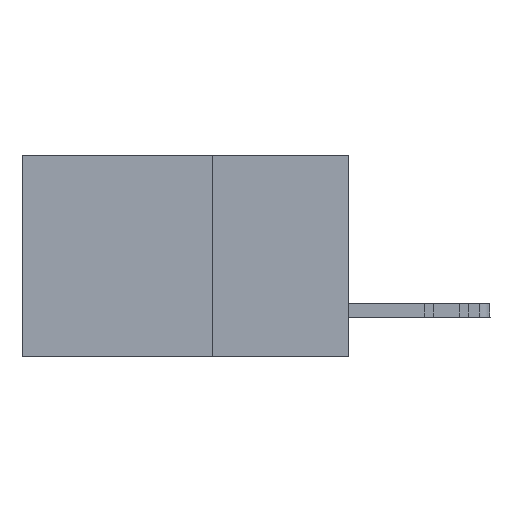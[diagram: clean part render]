
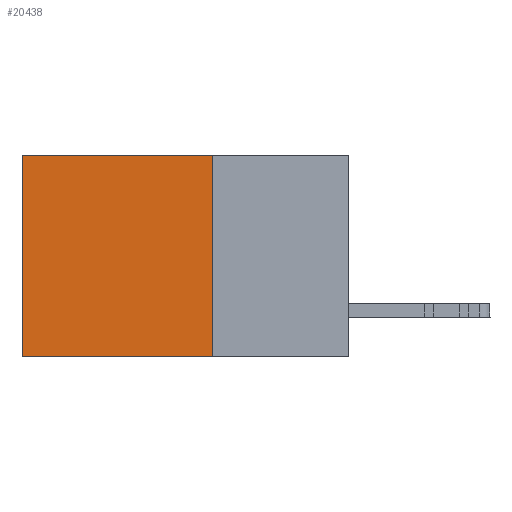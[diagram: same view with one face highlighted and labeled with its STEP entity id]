
A CAD part, left-side view. The second image highlights one B-rep face of the part: STEP entity #20438.
In plain terms, the highlighted planar face has unit normal (-1, 0, 0).
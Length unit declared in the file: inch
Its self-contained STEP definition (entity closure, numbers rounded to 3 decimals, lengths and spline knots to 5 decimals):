
#853 = ORIENTED_EDGE ( 'NONE', *, *, #7887, .F. ) ;
#2678 = VECTOR ( 'NONE', #27529, 39.37008 ) ;
#4890 = DIRECTION ( 'NONE',  ( 0., 0., -1. ) ) ;
#5564 = CARTESIAN_POINT ( 'NONE',  ( 0.298, 0.6, -0.37 ) ) ;
#6428 = VECTOR ( 'NONE', #21301, 39.37008 ) ;
#6734 = EDGE_CURVE ( 'NONE', #13923, #8608, #21188, .T. ) ;
#6937 = CARTESIAN_POINT ( 'NONE',  ( 0.298, 0.25, 0. ) ) ;
#7636 = VERTEX_POINT ( 'NONE', #16326 ) ;
#7887 = EDGE_CURVE ( 'NONE', #7636, #16645, #14452, .T. ) ;
#8142 = EDGE_CURVE ( 'NONE', #8608, #16645, #19667, .T. ) ;
#8325 = LINE ( 'NONE', #6937, #30068 ) ;
#8608 = VERTEX_POINT ( 'NONE', #23305 ) ;
#13923 = VERTEX_POINT ( 'NONE', #23910 ) ;
#14452 = LINE ( 'NONE', #25871, #25848 ) ;
#14478 = DIRECTION ( 'NONE',  ( 0., 1., 0. ) ) ;
#16326 = CARTESIAN_POINT ( 'NONE',  ( 0.298, 0.25, -0.37 ) ) ;
#16645 = VERTEX_POINT ( 'NONE', #5564 ) ;
#17936 = ORIENTED_EDGE ( 'NONE', *, *, #21636, .F. ) ;
#18665 = EDGE_LOOP ( 'NONE', ( #27851, #853, #17936, #24856 ) ) ;
#19285 = DIRECTION ( 'NONE',  ( 0., 0., -1. ) ) ;
#19667 = LINE ( 'NONE', #25021, #2678 ) ;
#20438 = ADVANCED_FACE ( 'NONE', ( #27948 ), #28565, .F. ) ;
#21188 = LINE ( 'NONE', #30538, #6428 ) ;
#21301 = DIRECTION ( 'NONE',  ( 0., 1., 0. ) ) ;
#21636 = EDGE_CURVE ( 'NONE', #13923, #7636, #8325, .T. ) ;
#23305 = CARTESIAN_POINT ( 'NONE',  ( 0.298, 0.6, 0. ) ) ;
#23864 = AXIS2_PLACEMENT_3D ( 'NONE', #28868, #26180, #19285 ) ;
#23910 = CARTESIAN_POINT ( 'NONE',  ( 0.298, 0.25, 0. ) ) ;
#24856 = ORIENTED_EDGE ( 'NONE', *, *, #6734, .T. ) ;
#25021 = CARTESIAN_POINT ( 'NONE',  ( 0.298, 0.6, 0. ) ) ;
#25848 = VECTOR ( 'NONE', #14478, 39.37008 ) ;
#25871 = CARTESIAN_POINT ( 'NONE',  ( 0.298, 0.25, -0.37 ) ) ;
#26180 = DIRECTION ( 'NONE',  ( 1., 0., 0. ) ) ;
#27529 = DIRECTION ( 'NONE',  ( 0., 0., -1. ) ) ;
#27851 = ORIENTED_EDGE ( 'NONE', *, *, #8142, .T. ) ;
#27948 = FACE_OUTER_BOUND ( 'NONE', #18665, .T. ) ;
#28565 = PLANE ( 'NONE',  #23864 ) ;
#28868 = CARTESIAN_POINT ( 'NONE',  ( 0.298, 0.25, 0. ) ) ;
#30068 = VECTOR ( 'NONE', #4890, 39.37008 ) ;
#30538 = CARTESIAN_POINT ( 'NONE',  ( 0.298, 0.25, 0. ) ) ;
